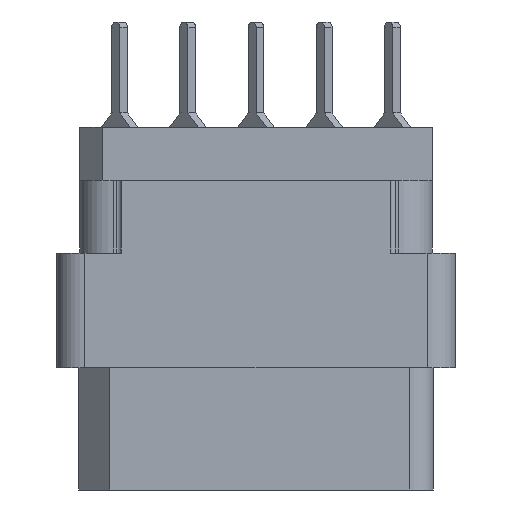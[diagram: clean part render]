
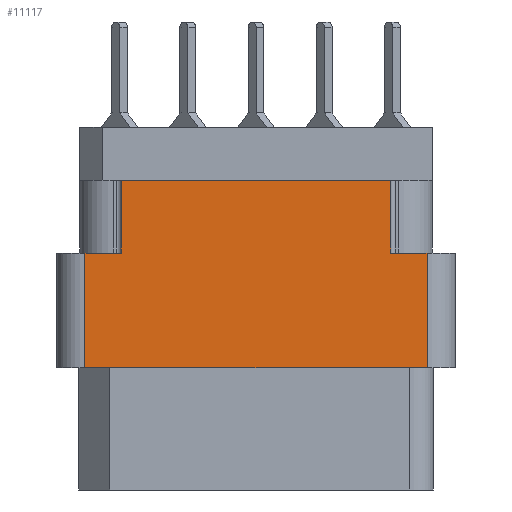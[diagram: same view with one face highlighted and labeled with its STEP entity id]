
A CAD part, left-side view. The second image highlights one B-rep face of the part: STEP entity #11117.
In plain terms, the highlighted planar face has unit normal (-1, 0, 0).
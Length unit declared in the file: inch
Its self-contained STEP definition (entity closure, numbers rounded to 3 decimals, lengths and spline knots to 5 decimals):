
#166 = ORIENTED_EDGE ( 'NONE', *, *, #28264, .F. ) ;
#559 = VECTOR ( 'NONE', #15948, 39.37008 ) ;
#959 = CARTESIAN_POINT ( 'NONE',  ( -1., 0.296, -0.117 ) ) ;
#1409 = LINE ( 'NONE', #30983, #23168 ) ;
#1447 = VERTEX_POINT ( 'NONE', #8112 ) ;
#1475 = DIRECTION ( 'NONE',  ( 0., 0., 1. ) ) ;
#1729 = DIRECTION ( 'NONE',  ( 0., 0., 1. ) ) ;
#2351 = VERTEX_POINT ( 'NONE', #32126 ) ;
#2641 = CARTESIAN_POINT ( 'NONE',  ( -1., -0.376, -0.277 ) ) ;
#2989 = VERTEX_POINT ( 'NONE', #17583 ) ;
#3050 = CARTESIAN_POINT ( 'NONE',  ( -1., 0.438, -0.277 ) ) ;
#3335 = LINE ( 'NONE', #20042, #25911 ) ;
#3351 = CARTESIAN_POINT ( 'NONE',  ( -1., -0.296, -0.277 ) ) ;
#3704 = DIRECTION ( 'NONE',  ( 0., 0., 1. ) ) ;
#3966 = ORIENTED_EDGE ( 'NONE', *, *, #23137, .T. ) ;
#4348 = DIRECTION ( 'NONE',  ( 0., 0., 1. ) ) ;
#4535 = DIRECTION ( 'NONE',  ( 0., -1., 0. ) ) ;
#5084 = VERTEX_POINT ( 'NONE', #8206 ) ;
#5566 = EDGE_LOOP ( 'NONE', ( #25153, #19822, #7960, #21205, #3966, #166, #21331, #12071 ) ) ;
#6800 = CARTESIAN_POINT ( 'NONE',  ( -1., -0.376, -0.798 ) ) ;
#7380 = EDGE_CURVE ( 'NONE', #2351, #9552, #9581, .T. ) ;
#7960 = ORIENTED_EDGE ( 'NONE', *, *, #7380, .T. ) ;
#8112 = CARTESIAN_POINT ( 'NONE',  ( -1., -0.296, -0.117 ) ) ;
#8206 = CARTESIAN_POINT ( 'NONE',  ( -1., 0.296, -0.277 ) ) ;
#9552 = VERTEX_POINT ( 'NONE', #2641 ) ;
#9581 = LINE ( 'NONE', #6800, #27065 ) ;
#11117 = ADVANCED_FACE ( 'NONE', ( #14236 ), #24044, .T. ) ;
#11616 = CARTESIAN_POINT ( 'NONE',  ( -1., -0.376, -0.798 ) ) ;
#11870 = CARTESIAN_POINT ( 'NONE',  ( -1., 0.438, -0.117 ) ) ;
#12071 = ORIENTED_EDGE ( 'NONE', *, *, #17153, .F. ) ;
#12216 = CARTESIAN_POINT ( 'NONE',  ( -1., 0.376, -0.529 ) ) ;
#13106 = EDGE_CURVE ( 'NONE', #25270, #2989, #1409, .T. ) ;
#13198 = DIRECTION ( 'NONE',  ( 0., -1., 0. ) ) ;
#14236 = FACE_OUTER_BOUND ( 'NONE', #5566, .T. ) ;
#15948 = DIRECTION ( 'NONE',  ( 0., 0., 1. ) ) ;
#16531 = DIRECTION ( 'NONE',  ( -1., 0., 0. ) ) ;
#16618 = LINE ( 'NONE', #11870, #17443 ) ;
#17153 = EDGE_CURVE ( 'NONE', #2989, #5084, #25460, .T. ) ;
#17443 = VECTOR ( 'NONE', #24617, 39.37008 ) ;
#17583 = CARTESIAN_POINT ( 'NONE',  ( -1., 0.376, -0.277 ) ) ;
#18398 = VERTEX_POINT ( 'NONE', #23177 ) ;
#18521 = EDGE_CURVE ( 'NONE', #5084, #32201, #19071, .T. ) ;
#18872 = EDGE_CURVE ( 'NONE', #2351, #25270, #3335, .T. ) ;
#18895 = LINE ( 'NONE', #3351, #559 ) ;
#19071 = LINE ( 'NONE', #29029, #32109 ) ;
#19584 = LINE ( 'NONE', #19904, #22988 ) ;
#19822 = ORIENTED_EDGE ( 'NONE', *, *, #18872, .F. ) ;
#19904 = CARTESIAN_POINT ( 'NONE',  ( -1., -0.296, -0.277 ) ) ;
#20042 = CARTESIAN_POINT ( 'NONE',  ( -1., -0.376, -0.529 ) ) ;
#21205 = ORIENTED_EDGE ( 'NONE', *, *, #24117, .F. ) ;
#21331 = ORIENTED_EDGE ( 'NONE', *, *, #18521, .F. ) ;
#22988 = VECTOR ( 'NONE', #4535, 39.37008 ) ;
#23137 = EDGE_CURVE ( 'NONE', #18398, #1447, #18895, .T. ) ;
#23168 = VECTOR ( 'NONE', #3704, 39.37008 ) ;
#23177 = CARTESIAN_POINT ( 'NONE',  ( -1., -0.296, -0.277 ) ) ;
#24044 = PLANE ( 'NONE',  #29656 ) ;
#24117 = EDGE_CURVE ( 'NONE', #18398, #9552, #19584, .T. ) ;
#24617 = DIRECTION ( 'NONE',  ( 0., -1., 0. ) ) ;
#25108 = DIRECTION ( 'NONE',  ( 0., 1., 0. ) ) ;
#25153 = ORIENTED_EDGE ( 'NONE', *, *, #13106, .F. ) ;
#25270 = VERTEX_POINT ( 'NONE', #12216 ) ;
#25460 = LINE ( 'NONE', #3050, #25890 ) ;
#25890 = VECTOR ( 'NONE', #13198, 39.37008 ) ;
#25911 = VECTOR ( 'NONE', #25108, 39.37008 ) ;
#27065 = VECTOR ( 'NONE', #4348, 39.37008 ) ;
#28264 = EDGE_CURVE ( 'NONE', #32201, #1447, #16618, .T. ) ;
#29029 = CARTESIAN_POINT ( 'NONE',  ( -1., 0.296, -0.277 ) ) ;
#29656 = AXIS2_PLACEMENT_3D ( 'NONE', #11616, #16531, #1475 ) ;
#30983 = CARTESIAN_POINT ( 'NONE',  ( -1., 0.376, -0.798 ) ) ;
#32109 = VECTOR ( 'NONE', #1729, 39.37008 ) ;
#32126 = CARTESIAN_POINT ( 'NONE',  ( -1., -0.376, -0.529 ) ) ;
#32201 = VERTEX_POINT ( 'NONE', #959 ) ;
